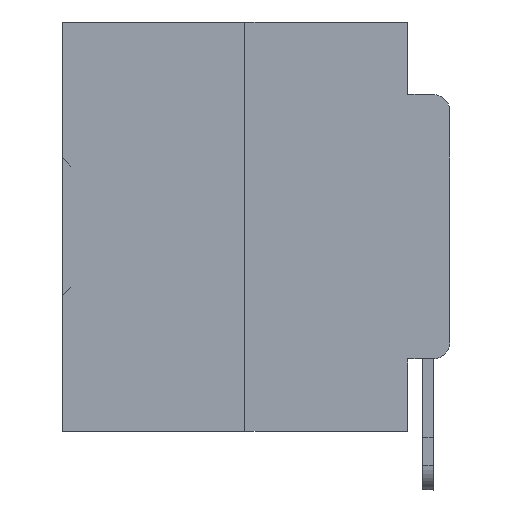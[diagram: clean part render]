
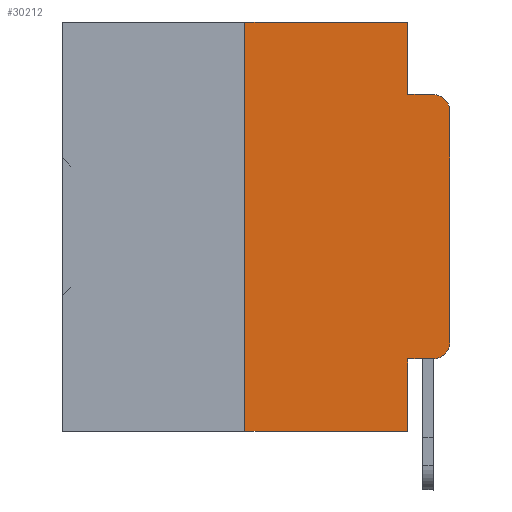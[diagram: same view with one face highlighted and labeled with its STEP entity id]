
A CAD part, left-side view. The second image highlights one B-rep face of the part: STEP entity #30212.
In plain terms, the highlighted planar face has unit normal (-1, 0, 0).
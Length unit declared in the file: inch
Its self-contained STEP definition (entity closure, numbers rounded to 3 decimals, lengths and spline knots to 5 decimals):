
#554 = DIRECTION ( 'NONE',  ( -1., 0., 0. ) ) ;
#623 = DIRECTION ( 'NONE',  ( 0., -1., 0. ) ) ;
#1033 = LINE ( 'NONE', #15865, #5637 ) ;
#1511 = DIRECTION ( 'NONE',  ( 0., -1., 0. ) ) ;
#1620 = LINE ( 'NONE', #35488, #34714 ) ;
#1801 = ORIENTED_EDGE ( 'NONE', *, *, #28913, .T. ) ;
#2276 = CARTESIAN_POINT ( 'NONE',  ( 0., 0.02, -0.0885 ) ) ;
#2520 = CIRCLE ( 'NONE', #6385, 0.02 ) ;
#2643 = VECTOR ( 'NONE', #6461, 39.37008 ) ;
#3061 = CARTESIAN_POINT ( 'NONE',  ( 0., 0.473, 0. ) ) ;
#5637 = VECTOR ( 'NONE', #623, 39.37008 ) ;
#6385 = AXIS2_PLACEMENT_3D ( 'NONE', #21075, #36528, #36736 ) ;
#6461 = DIRECTION ( 'NONE',  ( 0., -1., 0. ) ) ;
#6555 = DIRECTION ( 'NONE',  ( 0., 0., 1. ) ) ;
#6592 = EDGE_CURVE ( 'NONE', #28323, #18974, #13773, .T. ) ;
#7449 = DIRECTION ( 'NONE',  ( 0., 0., -1. ) ) ;
#8897 = DIRECTION ( 'NONE',  ( 0., 0., -1. ) ) ;
#9031 = DIRECTION ( 'NONE',  ( 0., 0., -1. ) ) ;
#10909 = VECTOR ( 'NONE', #6555, 39.37008 ) ;
#11962 = VERTEX_POINT ( 'NONE', #29850 ) ;
#12089 = LINE ( 'NONE', #3061, #2643 ) ;
#12341 = FACE_OUTER_BOUND ( 'NONE', #16081, .T. ) ;
#12690 = EDGE_CURVE ( 'NONE', #28323, #11962, #34976, .T. ) ;
#13356 = EDGE_CURVE ( 'NONE', #11962, #35758, #26982, .T. ) ;
#13624 = CARTESIAN_POINT ( 'NONE',  ( 0., 0.051, 0. ) ) ;
#13672 = CARTESIAN_POINT ( 'NONE',  ( 0., 0., -0.1085 ) ) ;
#13773 = LINE ( 'NONE', #17154, #20397 ) ;
#15141 = CARTESIAN_POINT ( 'NONE',  ( 0., 0.051, -0.5 ) ) ;
#15865 = CARTESIAN_POINT ( 'NONE',  ( 0., 0.473, -0.5 ) ) ;
#16081 = EDGE_LOOP ( 'NONE', ( #25066, #1801, #28372, #34534, #21314, #17327, #22864, #37487, #25555, #21117 ) ) ;
#16706 = VECTOR ( 'NONE', #1511, 39.37008 ) ;
#16850 = DIRECTION ( 'NONE',  ( 0., -1., 0. ) ) ;
#17154 = CARTESIAN_POINT ( 'NONE',  ( 0., 0.051, 0. ) ) ;
#17327 = ORIENTED_EDGE ( 'NONE', *, *, #29922, .F. ) ;
#18566 = EDGE_CURVE ( 'NONE', #39117, #32693, #1620, .T. ) ;
#18974 = VERTEX_POINT ( 'NONE', #15141 ) ;
#19472 = EDGE_CURVE ( 'NONE', #35758, #26736, #31081, .T. ) ;
#20397 = VECTOR ( 'NONE', #29381, 39.37008 ) ;
#21075 = CARTESIAN_POINT ( 'NONE',  ( 0., 0.02, -0.1085 ) ) ;
#21117 = ORIENTED_EDGE ( 'NONE', *, *, #13356, .T. ) ;
#21314 = ORIENTED_EDGE ( 'NONE', *, *, #36322, .F. ) ;
#21420 = CARTESIAN_POINT ( 'NONE',  ( 0., 0.25, -0.5 ) ) ;
#22262 = DIRECTION ( 'NONE',  ( 1., 0., 0. ) ) ;
#22864 = ORIENTED_EDGE ( 'NONE', *, *, #27814, .T. ) ;
#23355 = CARTESIAN_POINT ( 'NONE',  ( 0., 0.25, 0. ) ) ;
#23544 = CARTESIAN_POINT ( 'NONE',  ( 0., 0.051, -0.4115 ) ) ;
#23883 = VERTEX_POINT ( 'NONE', #21420 ) ;
#24795 = CARTESIAN_POINT ( 'NONE',  ( 0., 0.25, 0. ) ) ;
#25066 = ORIENTED_EDGE ( 'NONE', *, *, #19472, .T. ) ;
#25555 = ORIENTED_EDGE ( 'NONE', *, *, #12690, .T. ) ;
#26529 = CARTESIAN_POINT ( 'NONE',  ( 0., 0.051, -0.0885 ) ) ;
#26736 = VERTEX_POINT ( 'NONE', #13672 ) ;
#26982 = CIRCLE ( 'NONE', #32119, 0.02 ) ;
#27814 = EDGE_CURVE ( 'NONE', #23883, #18974, #1033, .T. ) ;
#27880 = DIRECTION ( 'NONE',  ( 0., 0., 1. ) ) ;
#28226 = AXIS2_PLACEMENT_3D ( 'NONE', #28307, #22262, #7449 ) ;
#28307 = CARTESIAN_POINT ( 'NONE',  ( 0., 0.473, 0. ) ) ;
#28323 = VERTEX_POINT ( 'NONE', #23544 ) ;
#28372 = ORIENTED_EDGE ( 'NONE', *, *, #18566, .F. ) ;
#28477 = EDGE_CURVE ( 'NONE', #31746, #39117, #36364, .T. ) ;
#28619 = CARTESIAN_POINT ( 'NONE',  ( 0., 0.02, -0.3915 ) ) ;
#28907 = PLANE ( 'NONE',  #28226 ) ;
#28913 = EDGE_CURVE ( 'NONE', #26736, #32693, #2520, .T. ) ;
#29381 = DIRECTION ( 'NONE',  ( 0., 0., -1. ) ) ;
#29650 = VECTOR ( 'NONE', #27880, 39.37008 ) ;
#29850 = CARTESIAN_POINT ( 'NONE',  ( 0., 0.02, -0.4115 ) ) ;
#29922 = EDGE_CURVE ( 'NONE', #23883, #38632, #37816, .T. ) ;
#30212 = ADVANCED_FACE ( 'NONE', ( #12341 ), #28907, .F. ) ;
#30971 = CARTESIAN_POINT ( 'NONE',  ( 0., 0.051, 0. ) ) ;
#31081 = LINE ( 'NONE', #37477, #29650 ) ;
#31746 = VERTEX_POINT ( 'NONE', #13624 ) ;
#31781 = CARTESIAN_POINT ( 'NONE',  ( 0., 0.051, -0.4115 ) ) ;
#32119 = AXIS2_PLACEMENT_3D ( 'NONE', #28619, #554, #9031 ) ;
#32611 = VECTOR ( 'NONE', #8897, 39.37008 ) ;
#32693 = VERTEX_POINT ( 'NONE', #2276 ) ;
#34534 = ORIENTED_EDGE ( 'NONE', *, *, #28477, .F. ) ;
#34714 = VECTOR ( 'NONE', #16850, 39.37008 ) ;
#34976 = LINE ( 'NONE', #31781, #16706 ) ;
#35427 = CARTESIAN_POINT ( 'NONE',  ( 0., 0., -0.3915 ) ) ;
#35488 = CARTESIAN_POINT ( 'NONE',  ( 0., 0.051, -0.0885 ) ) ;
#35758 = VERTEX_POINT ( 'NONE', #35427 ) ;
#36322 = EDGE_CURVE ( 'NONE', #38632, #31746, #12089, .T. ) ;
#36364 = LINE ( 'NONE', #30971, #32611 ) ;
#36528 = DIRECTION ( 'NONE',  ( -1., 0., 0. ) ) ;
#36736 = DIRECTION ( 'NONE',  ( 0., 0., -1. ) ) ;
#37477 = CARTESIAN_POINT ( 'NONE',  ( 0., 0., 0. ) ) ;
#37487 = ORIENTED_EDGE ( 'NONE', *, *, #6592, .F. ) ;
#37816 = LINE ( 'NONE', #24795, #10909 ) ;
#38632 = VERTEX_POINT ( 'NONE', #23355 ) ;
#39117 = VERTEX_POINT ( 'NONE', #26529 ) ;
